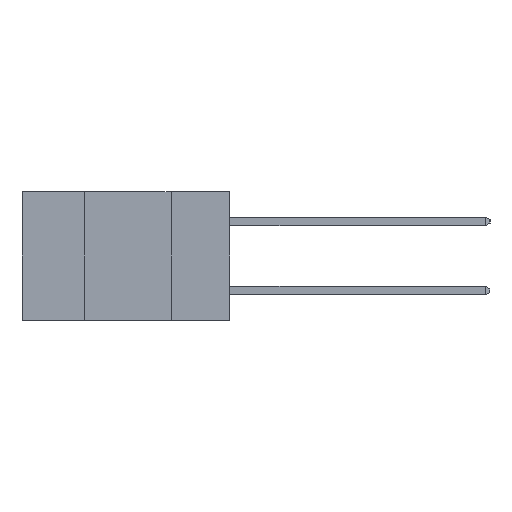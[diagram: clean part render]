
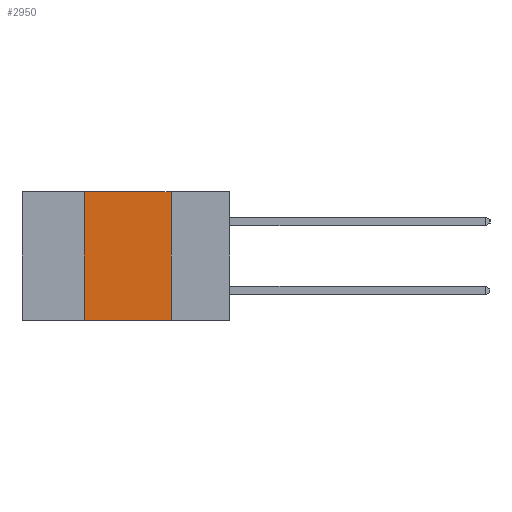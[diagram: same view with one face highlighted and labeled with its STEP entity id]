
A CAD part, left-side view. The second image highlights one B-rep face of the part: STEP entity #2950.
In plain terms, the highlighted planar face has unit normal (-1, 0, 0).
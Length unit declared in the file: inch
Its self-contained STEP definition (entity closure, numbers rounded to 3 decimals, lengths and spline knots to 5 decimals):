
#210 = CARTESIAN_POINT ( 'NONE',  ( 0., 0.17, 0. ) ) ;
#572 = CARTESIAN_POINT ( 'NONE',  ( 0., 0.17, -0.37 ) ) ;
#606 = VECTOR ( 'NONE', #12510, 39.37008 ) ;
#1016 = LINE ( 'NONE', #2094, #3455 ) ;
#1713 = VERTEX_POINT ( 'NONE', #210 ) ;
#1748 = VECTOR ( 'NONE', #2572, 39.37008 ) ;
#1767 = EDGE_CURVE ( 'NONE', #9015, #7716, #13208, .T. ) ;
#1891 = EDGE_LOOP ( 'NONE', ( #11352, #3631, #6070, #7927 ) ) ;
#2094 = CARTESIAN_POINT ( 'NONE',  ( 0., 0.42, 0. ) ) ;
#2115 = FACE_OUTER_BOUND ( 'NONE', #1891, .T. ) ;
#2572 = DIRECTION ( 'NONE',  ( 0., 0., -1. ) ) ;
#2950 = ADVANCED_FACE ( 'NONE', ( #2115 ), #10914, .F. ) ;
#3238 = CARTESIAN_POINT ( 'NONE',  ( 0., 0.6, 0. ) ) ;
#3455 = VECTOR ( 'NONE', #3636, 39.37008 ) ;
#3631 = ORIENTED_EDGE ( 'NONE', *, *, #6013, .F. ) ;
#3636 = DIRECTION ( 'NONE',  ( 0., 0., 1. ) ) ;
#4200 = EDGE_CURVE ( 'NONE', #9015, #8498, #1016, .T. ) ;
#5635 = LINE ( 'NONE', #12686, #1748 ) ;
#6013 = EDGE_CURVE ( 'NONE', #8498, #1713, #9887, .T. ) ;
#6070 = ORIENTED_EDGE ( 'NONE', *, *, #4200, .F. ) ;
#7239 = CARTESIAN_POINT ( 'NONE',  ( 0., 0.42, -0.37 ) ) ;
#7716 = VERTEX_POINT ( 'NONE', #572 ) ;
#7927 = ORIENTED_EDGE ( 'NONE', *, *, #1767, .T. ) ;
#8498 = VERTEX_POINT ( 'NONE', #9929 ) ;
#9015 = VERTEX_POINT ( 'NONE', #7239 ) ;
#9031 = CARTESIAN_POINT ( 'NONE',  ( 0., 0.6, -0.37 ) ) ;
#9887 = LINE ( 'NONE', #10816, #606 ) ;
#9929 = CARTESIAN_POINT ( 'NONE',  ( 0., 0.42, 0. ) ) ;
#10294 = EDGE_CURVE ( 'NONE', #1713, #7716, #5635, .T. ) ;
#10457 = DIRECTION ( 'NONE',  ( 1., 0., 0. ) ) ;
#10816 = CARTESIAN_POINT ( 'NONE',  ( 0., 0.6, 0. ) ) ;
#10914 = PLANE ( 'NONE',  #12316 ) ;
#11195 = DIRECTION ( 'NONE',  ( 0., 0., -1. ) ) ;
#11352 = ORIENTED_EDGE ( 'NONE', *, *, #10294, .F. ) ;
#12004 = DIRECTION ( 'NONE',  ( 0., -1., 0. ) ) ;
#12316 = AXIS2_PLACEMENT_3D ( 'NONE', #3238, #10457, #11195 ) ;
#12510 = DIRECTION ( 'NONE',  ( 0., -1., 0. ) ) ;
#12686 = CARTESIAN_POINT ( 'NONE',  ( 0., 0.17, 0. ) ) ;
#12895 = VECTOR ( 'NONE', #12004, 39.37008 ) ;
#13208 = LINE ( 'NONE', #9031, #12895 ) ;
